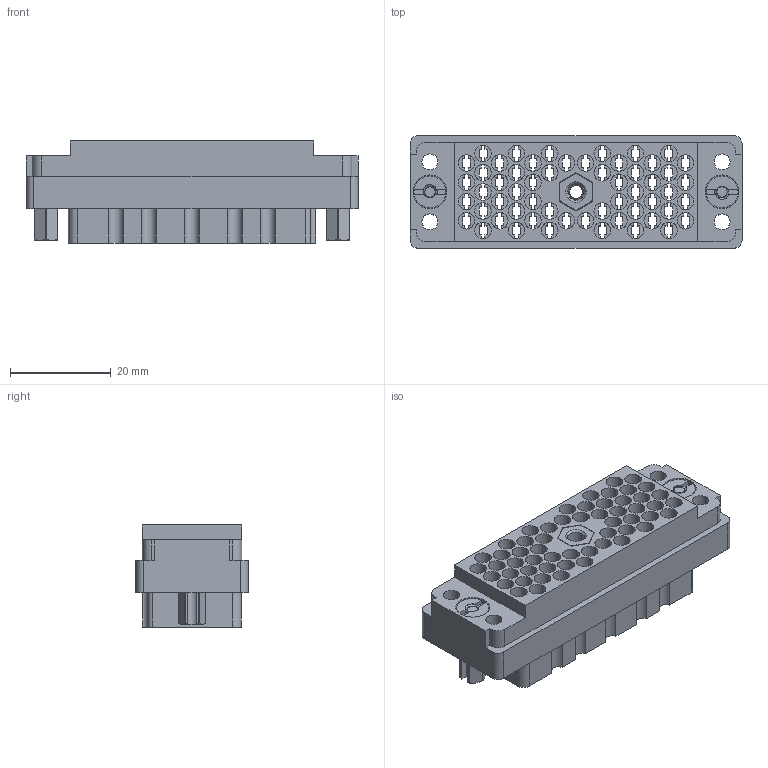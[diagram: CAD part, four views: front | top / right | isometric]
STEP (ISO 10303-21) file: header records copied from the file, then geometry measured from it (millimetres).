
FILE_DESCRIPTION (( 'STEP AP203' ), '1' );
FILE_NAME ('516-056-000-202.STEP', '2020-03-05T19:19:01', ( '' ), ( '' ), 'SwSTEP 2.0', 'SolidWorks 2016', '' );
FILE_SCHEMA (( 'CONFIG_CONTROL_DESIGN' ));
Length unit declared in the file: inch
Products named in the file (6): 516-221-038-102_057; 516-252-035-100_516-252-035-100; 516-056-000-202; 516-221-038-102_056; 516-252-021-102_056; 516 Part Receptacle_056
Assembly tree (6 placements, depth 2):
  516-056-000-202
    516 Part Receptacle_056
    516-252-021-102_056  x2
    516-221-038-102_056
    516-252-035-100_516-252-035-100
    516-221-038-102_057
Bounding box: 65.84 x 22.25 x 20.27 mm (x, y, z)
Volume: 14583.4 mm3; surface area: 21126.9 mm2
Topology: 6 solids, 6 shells, 1486 faces, 4332 edges, 2874 vertices
Faces by surface type: plane 951, cylinder 457, cone 44, bspline 34
Entity records: 55394 total; most frequent: CARTESIAN_POINT 15512, ORIENTED_EDGE 8476, DIRECTION 7994, EDGE_CURVE 4238, VECTOR 2926, LINE 2926, VERTEX_POINT 2814, AXIS2_PLACEMENT_3D 2534
